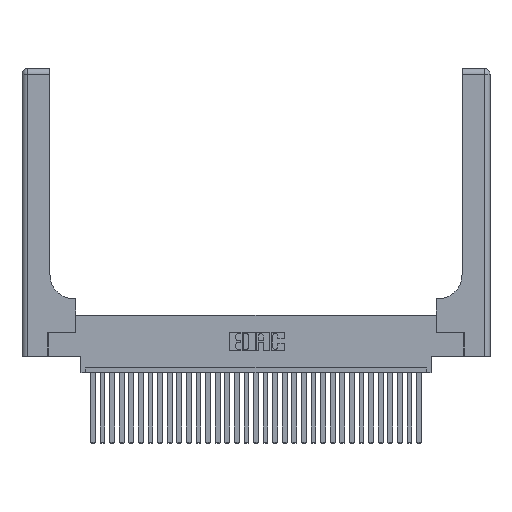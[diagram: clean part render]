
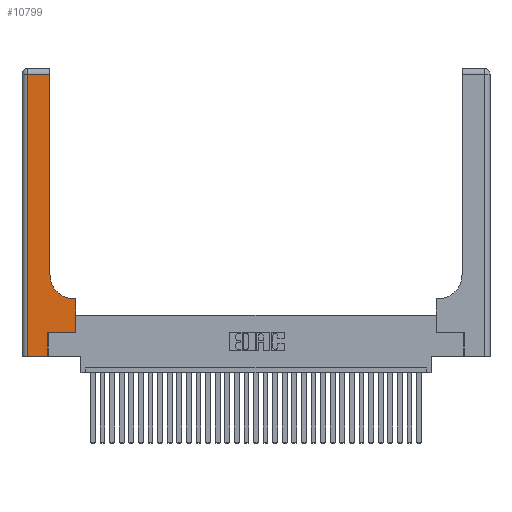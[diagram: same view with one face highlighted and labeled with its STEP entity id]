
A CAD part, top view. The second image highlights one B-rep face of the part: STEP entity #10799.
In plain terms, the highlighted planar face has unit normal (0, 0, 1).
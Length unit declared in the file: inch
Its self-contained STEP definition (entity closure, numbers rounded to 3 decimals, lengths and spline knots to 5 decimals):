
#295 = ORIENTED_EDGE ( 'NONE', *, *, #15642, .T. ) ;
#409 = LINE ( 'NONE', #1956, #27154 ) ;
#1271 = VERTEX_POINT ( 'NONE', #29646 ) ;
#1577 = DIRECTION ( 'NONE',  ( 0., 0., -1. ) ) ;
#1903 = CARTESIAN_POINT ( 'NONE',  ( 0.5415, 0.85, 0.37 ) ) ;
#1956 = CARTESIAN_POINT ( 'NONE',  ( 0.5585, 0.25, 0.37 ) ) ;
#2036 = VECTOR ( 'NONE', #23619, 39.37008 ) ;
#2319 = CARTESIAN_POINT ( 'NONE',  ( 0.2915, 0.6, 0.37 ) ) ;
#2622 = VERTEX_POINT ( 'NONE', #32306 ) ;
#3316 = ORIENTED_EDGE ( 'NONE', *, *, #25106, .T. ) ;
#3870 = DIRECTION ( 'NONE',  ( 0., 0., -1. ) ) ;
#5118 = VECTOR ( 'NONE', #25999, 39.37008 ) ;
#5248 = ORIENTED_EDGE ( 'NONE', *, *, #13170, .T. ) ;
#5268 = VECTOR ( 'NONE', #31538, 39.37008 ) ;
#6091 = LINE ( 'NONE', #2319, #28038 ) ;
#6176 = CARTESIAN_POINT ( 'NONE',  ( 0.269, 0., 0.37 ) ) ;
#6752 = LINE ( 'NONE', #6176, #5118 ) ;
#7038 = VECTOR ( 'NONE', #17703, 39.37008 ) ;
#7100 = VERTEX_POINT ( 'NONE', #23457 ) ;
#7105 = DIRECTION ( 'NONE',  ( 1., 0., 0. ) ) ;
#7534 = DIRECTION ( 'NONE',  ( -1., 0., 0. ) ) ;
#9420 = FACE_OUTER_BOUND ( 'NONE', #13486, .T. ) ;
#9448 = EDGE_CURVE ( 'NONE', #26127, #17676, #409, .T. ) ;
#9596 = EDGE_CURVE ( 'NONE', #1271, #31263, #27873, .T. ) ;
#9984 = VERTEX_POINT ( 'NONE', #14125 ) ;
#10754 = DIRECTION ( 'NONE',  ( 0., 1., 0. ) ) ;
#10799 = ADVANCED_FACE ( 'NONE', ( #9420 ), #21638, .F. ) ;
#11445 = ORIENTED_EDGE ( 'NONE', *, *, #9448, .T. ) ;
#11583 = EDGE_CURVE ( 'NONE', #12769, #7100, #6752, .T. ) ;
#11977 = EDGE_CURVE ( 'NONE', #9984, #1271, #14499, .T. ) ;
#12015 = LINE ( 'NONE', #18766, #5268 ) ;
#12769 = VERTEX_POINT ( 'NONE', #21918 ) ;
#13170 = EDGE_CURVE ( 'NONE', #31263, #14179, #13593, .T. ) ;
#13384 = LINE ( 'NONE', #23470, #17657 ) ;
#13486 = EDGE_LOOP ( 'NONE', ( #14316, #30084, #5248, #295, #16348, #19695, #11445, #14696, #3316 ) ) ;
#13593 = LINE ( 'NONE', #19433, #30351 ) ;
#13634 = CIRCLE ( 'NONE', #22745, 0.25 ) ;
#14125 = CARTESIAN_POINT ( 'NONE',  ( 0.2915, 0.85, 0.37 ) ) ;
#14179 = VERTEX_POINT ( 'NONE', #28023 ) ;
#14316 = ORIENTED_EDGE ( 'NONE', *, *, #11977, .T. ) ;
#14499 = LINE ( 'NONE', #22936, #7038 ) ;
#14696 = ORIENTED_EDGE ( 'NONE', *, *, #18464, .T. ) ;
#15642 = EDGE_CURVE ( 'NONE', #14179, #12769, #13384, .T. ) ;
#16348 = ORIENTED_EDGE ( 'NONE', *, *, #11583, .T. ) ;
#17657 = VECTOR ( 'NONE', #18430, 39.37008 ) ;
#17676 = VERTEX_POINT ( 'NONE', #26001 ) ;
#17703 = DIRECTION ( 'NONE',  ( 0., 1., 0. ) ) ;
#18430 = DIRECTION ( 'NONE',  ( 1., 0., 0. ) ) ;
#18464 = EDGE_CURVE ( 'NONE', #17676, #2622, #6091, .T. ) ;
#18645 = CARTESIAN_POINT ( 'NONE',  ( 0.06, 2.94, 0.37 ) ) ;
#18766 = CARTESIAN_POINT ( 'NONE',  ( 0.269, 0.25, 0.37 ) ) ;
#19433 = CARTESIAN_POINT ( 'NONE',  ( 0.06, 3., 0.37 ) ) ;
#19695 = ORIENTED_EDGE ( 'NONE', *, *, #31341, .T. ) ;
#20962 = CARTESIAN_POINT ( 'NONE',  ( 0., 2.94, 0.37 ) ) ;
#21638 = PLANE ( 'NONE',  #22179 ) ;
#21918 = CARTESIAN_POINT ( 'NONE',  ( 0.269, 0., 0.37 ) ) ;
#22179 = AXIS2_PLACEMENT_3D ( 'NONE', #31275, #3870, #27527 ) ;
#22745 = AXIS2_PLACEMENT_3D ( 'NONE', #1903, #1577, #7105 ) ;
#22936 = CARTESIAN_POINT ( 'NONE',  ( 0.2915, 3., 0.37 ) ) ;
#23457 = CARTESIAN_POINT ( 'NONE',  ( 0.269, 0.25, 0.37 ) ) ;
#23470 = CARTESIAN_POINT ( 'NONE',  ( 0., 0., 0.37 ) ) ;
#23619 = DIRECTION ( 'NONE',  ( -1., 0., 0. ) ) ;
#25106 = EDGE_CURVE ( 'NONE', #2622, #9984, #13634, .T. ) ;
#25999 = DIRECTION ( 'NONE',  ( 0., 1., 0. ) ) ;
#26001 = CARTESIAN_POINT ( 'NONE',  ( 0.5585, 0.6, 0.37 ) ) ;
#26127 = VERTEX_POINT ( 'NONE', #30918 ) ;
#27154 = VECTOR ( 'NONE', #10754, 39.37008 ) ;
#27527 = DIRECTION ( 'NONE',  ( -1., 0., 0. ) ) ;
#27873 = LINE ( 'NONE', #20962, #2036 ) ;
#28023 = CARTESIAN_POINT ( 'NONE',  ( 0.06, 0., 0.37 ) ) ;
#28038 = VECTOR ( 'NONE', #7534, 39.37008 ) ;
#29646 = CARTESIAN_POINT ( 'NONE',  ( 0.2915, 2.94, 0.37 ) ) ;
#30084 = ORIENTED_EDGE ( 'NONE', *, *, #9596, .T. ) ;
#30351 = VECTOR ( 'NONE', #31995, 39.37008 ) ;
#30918 = CARTESIAN_POINT ( 'NONE',  ( 0.5585, 0.25, 0.37 ) ) ;
#31263 = VERTEX_POINT ( 'NONE', #18645 ) ;
#31275 = CARTESIAN_POINT ( 'NONE',  ( 0., 3., 0.37 ) ) ;
#31341 = EDGE_CURVE ( 'NONE', #7100, #26127, #12015, .T. ) ;
#31538 = DIRECTION ( 'NONE',  ( 1., 0., 0. ) ) ;
#31995 = DIRECTION ( 'NONE',  ( 0., -1., 0. ) ) ;
#32306 = CARTESIAN_POINT ( 'NONE',  ( 0.5415, 0.6, 0.37 ) ) ;
